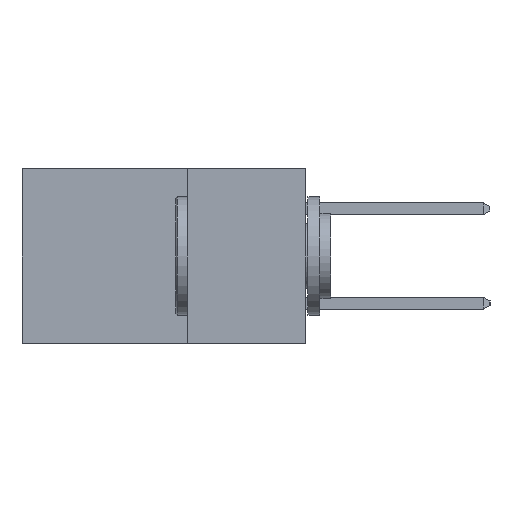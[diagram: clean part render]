
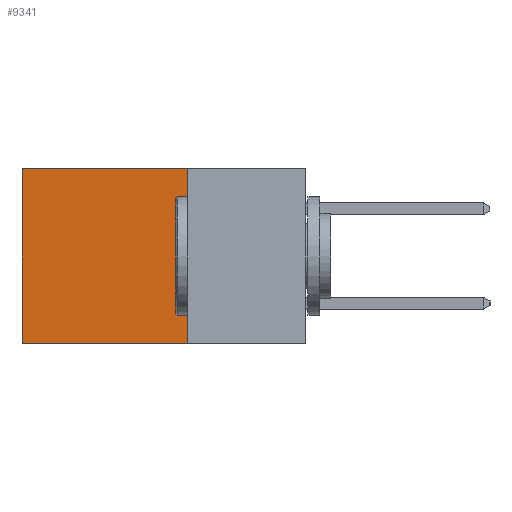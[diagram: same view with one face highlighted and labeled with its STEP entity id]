
A CAD part, left-side view. The second image highlights one B-rep face of the part: STEP entity #9341.
In plain terms, the highlighted planar face has unit normal (-1, 0, 0).
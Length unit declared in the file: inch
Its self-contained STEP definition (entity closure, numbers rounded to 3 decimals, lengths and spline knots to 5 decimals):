
#244 = CARTESIAN_POINT ( 'NONE',  ( 0.2615, 0.6, -0.37 ) ) ;
#308 = DIRECTION ( 'NONE',  ( 0., 0., -1. ) ) ;
#1196 = LINE ( 'NONE', #2182, #2801 ) ;
#1393 = VECTOR ( 'NONE', #2819, 39.37008 ) ;
#1397 = DIRECTION ( 'NONE',  ( 0., 1., 0. ) ) ;
#1907 = LINE ( 'NONE', #5978, #2162 ) ;
#2041 = DIRECTION ( 'NONE',  ( 0., 1., 0. ) ) ;
#2110 = ORIENTED_EDGE ( 'NONE', *, *, #6105, .T. ) ;
#2162 = VECTOR ( 'NONE', #308, 39.37008 ) ;
#2168 = CARTESIAN_POINT ( 'NONE',  ( 0.2615, 0.25, -0.37 ) ) ;
#2182 = CARTESIAN_POINT ( 'NONE',  ( 0.2615, 0.25, 0. ) ) ;
#2299 = ORIENTED_EDGE ( 'NONE', *, *, #8294, .F. ) ;
#2336 = ORIENTED_EDGE ( 'NONE', *, *, #7523, .F. ) ;
#2396 = VECTOR ( 'NONE', #1397, 39.37008 ) ;
#2801 = VECTOR ( 'NONE', #2041, 39.37008 ) ;
#2819 = DIRECTION ( 'NONE',  ( 0., 0., -1. ) ) ;
#2840 = CARTESIAN_POINT ( 'NONE',  ( 0.2615, 0.6, -0.37 ) ) ;
#3422 = EDGE_LOOP ( 'NONE', ( #2110, #2299, #2336, #6947 ) ) ;
#3553 = PLANE ( 'NONE',  #4079 ) ;
#4079 = AXIS2_PLACEMENT_3D ( 'NONE', #9059, #4395, #9786 ) ;
#4395 = DIRECTION ( 'NONE',  ( 1., 0., 0. ) ) ;
#4750 = EDGE_CURVE ( 'NONE', #6915, #8652, #1196, .T. ) ;
#5978 = CARTESIAN_POINT ( 'NONE',  ( 0.2615, 0.25, -0.37 ) ) ;
#6105 = EDGE_CURVE ( 'NONE', #8652, #6524, #6219, .T. ) ;
#6219 = LINE ( 'NONE', #2840, #1393 ) ;
#6524 = VERTEX_POINT ( 'NONE', #244 ) ;
#6696 = FACE_OUTER_BOUND ( 'NONE', #3422, .T. ) ;
#6915 = VERTEX_POINT ( 'NONE', #7819 ) ;
#6947 = ORIENTED_EDGE ( 'NONE', *, *, #4750, .T. ) ;
#7459 = CARTESIAN_POINT ( 'NONE',  ( 0.2615, 0.6, 0. ) ) ;
#7523 = EDGE_CURVE ( 'NONE', #6915, #7583, #1907, .T. ) ;
#7583 = VERTEX_POINT ( 'NONE', #9085 ) ;
#7819 = CARTESIAN_POINT ( 'NONE',  ( 0.2615, 0.25, 0. ) ) ;
#8294 = EDGE_CURVE ( 'NONE', #7583, #6524, #8722, .T. ) ;
#8652 = VERTEX_POINT ( 'NONE', #7459 ) ;
#8722 = LINE ( 'NONE', #2168, #2396 ) ;
#9059 = CARTESIAN_POINT ( 'NONE',  ( 0.2615, 0.25, -0.37 ) ) ;
#9085 = CARTESIAN_POINT ( 'NONE',  ( 0.2615, 0.25, -0.37 ) ) ;
#9341 = ADVANCED_FACE ( 'NONE', ( #6696 ), #3553, .F. ) ;
#9786 = DIRECTION ( 'NONE',  ( 0., 0., -1. ) ) ;
